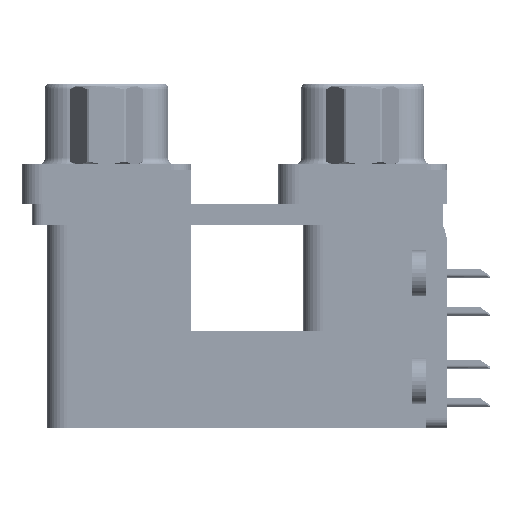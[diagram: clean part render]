
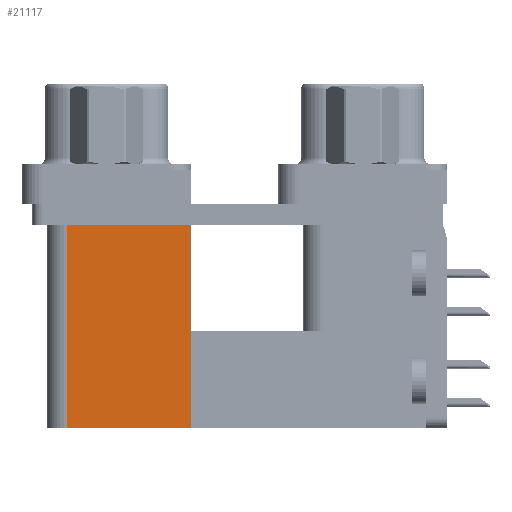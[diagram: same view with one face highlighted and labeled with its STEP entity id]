
A CAD part, left-side view. The second image highlights one B-rep face of the part: STEP entity #21117.
In plain terms, the highlighted planar face has unit normal (-1, 0, 0).
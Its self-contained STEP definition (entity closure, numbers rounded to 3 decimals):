
#641 = DIRECTION ( 'NONE',  ( 0., 1., 0. ) ) ;
#3027 = CARTESIAN_POINT ( 'NONE',  ( 3.7, 21.975, -19.2 ) ) ;
#4393 = ORIENTED_EDGE ( 'NONE', *, *, #17804, .F. ) ;
#6282 = EDGE_LOOP ( 'NONE', ( #12049, #24083, #4393, #40985 ) ) ;
#6378 = DIRECTION ( 'NONE',  ( 0., 1., 0. ) ) ;
#8531 = CARTESIAN_POINT ( 'NONE',  ( 3.7, 21.975, -2.5 ) ) ;
#8944 = VECTOR ( 'NONE', #22485, 1000. ) ;
#11197 = FACE_OUTER_BOUND ( 'NONE', #6282, .T. ) ;
#12049 = ORIENTED_EDGE ( 'NONE', *, *, #15259, .T. ) ;
#14595 = DIRECTION ( 'NONE',  ( 0., 1., 0. ) ) ;
#15259 = EDGE_CURVE ( 'NONE', #45326, #35144, #21725, .T. ) ;
#16024 = VECTOR ( 'NONE', #641, 1000. ) ;
#17011 = DIRECTION ( 'NONE',  ( 0., 0., 1. ) ) ;
#17242 = LINE ( 'NONE', #3027, #26790 ) ;
#17804 = EDGE_CURVE ( 'NONE', #27109, #26616, #47073, .T. ) ;
#18402 = CARTESIAN_POINT ( 'NONE',  ( 3.7, 12.775, -19.2 ) ) ;
#20192 = VECTOR ( 'NONE', #6378, 1000. ) ;
#21117 = ADVANCED_FACE ( 'NONE', ( #11197 ), #40574, .F. ) ;
#21725 = LINE ( 'NONE', #32535, #16024 ) ;
#22472 = EDGE_CURVE ( 'NONE', #27109, #45326, #33082, .T. ) ;
#22485 = DIRECTION ( 'NONE',  ( 0., 0., 1. ) ) ;
#24083 = ORIENTED_EDGE ( 'NONE', *, *, #26317, .F. ) ;
#26317 = EDGE_CURVE ( 'NONE', #26616, #35144, #17242, .T. ) ;
#26616 = VERTEX_POINT ( 'NONE', #33467 ) ;
#26790 = VECTOR ( 'NONE', #17011, 1000. ) ;
#27109 = VERTEX_POINT ( 'NONE', #28870 ) ;
#28870 = CARTESIAN_POINT ( 'NONE',  ( 3.7, 12.775, -19.2 ) ) ;
#32535 = CARTESIAN_POINT ( 'NONE',  ( 3.7, 12.775, -2.5 ) ) ;
#33082 = LINE ( 'NONE', #18402, #8944 ) ;
#33467 = CARTESIAN_POINT ( 'NONE',  ( 3.7, 21.975, -19.2 ) ) ;
#35144 = VERTEX_POINT ( 'NONE', #8531 ) ;
#40096 = CARTESIAN_POINT ( 'NONE',  ( 3.7, 12.775, -19.2 ) ) ;
#40337 = CARTESIAN_POINT ( 'NONE',  ( 3.7, 12.775, -19.2 ) ) ;
#40574 = PLANE ( 'NONE',  #45722 ) ;
#40985 = ORIENTED_EDGE ( 'NONE', *, *, #22472, .T. ) ;
#44189 = DIRECTION ( 'NONE',  ( 1., 0., 0. ) ) ;
#45326 = VERTEX_POINT ( 'NONE', #47127 ) ;
#45722 = AXIS2_PLACEMENT_3D ( 'NONE', #40337, #44189, #14595 ) ;
#47073 = LINE ( 'NONE', #40096, #20192 ) ;
#47127 = CARTESIAN_POINT ( 'NONE',  ( 3.7, 12.775, -2.5 ) ) ;
